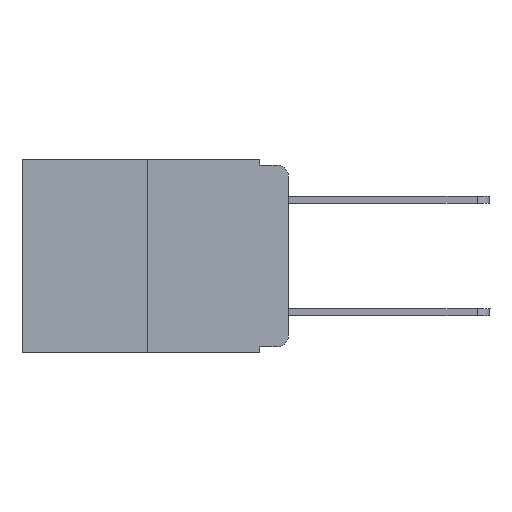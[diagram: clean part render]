
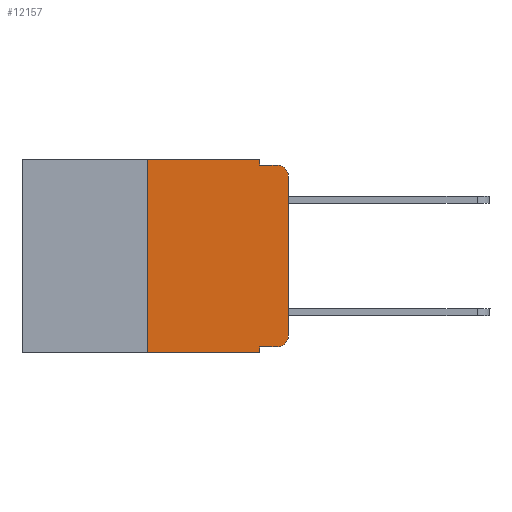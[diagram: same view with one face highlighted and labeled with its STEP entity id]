
A CAD part, left-side view. The second image highlights one B-rep face of the part: STEP entity #12157.
In plain terms, the highlighted planar face has unit normal (-1, 0, 0).
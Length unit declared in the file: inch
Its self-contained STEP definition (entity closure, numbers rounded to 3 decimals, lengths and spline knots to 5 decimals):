
#166 = LINE ( 'NONE', #14627, #7248 ) ;
#282 = EDGE_CURVE ( 'NONE', #3871, #5701, #5324, .T. ) ;
#373 = CARTESIAN_POINT ( 'NONE',  ( 0., 0.02, -0.313 ) ) ;
#478 = ORIENTED_EDGE ( 'NONE', *, *, #15215, .T. ) ;
#643 = VECTOR ( 'NONE', #9150, 39.37008 ) ;
#799 = DIRECTION ( 'NONE',  ( 0., 0., -1. ) ) ;
#820 = VERTEX_POINT ( 'NONE', #844 ) ;
#844 = CARTESIAN_POINT ( 'NONE',  ( 0., 0.02, -0.333 ) ) ;
#1194 = EDGE_CURVE ( 'NONE', #10381, #2462, #6404, .T. ) ;
#1381 = VERTEX_POINT ( 'NONE', #11010 ) ;
#1392 = ORIENTED_EDGE ( 'NONE', *, *, #11559, .T. ) ;
#1695 = DIRECTION ( 'NONE',  ( 0., 0., -1. ) ) ;
#1762 = VECTOR ( 'NONE', #799, 39.37008 ) ;
#2462 = VERTEX_POINT ( 'NONE', #12397 ) ;
#2502 = DIRECTION ( 'NONE',  ( 1., 0., 0. ) ) ;
#2758 = VERTEX_POINT ( 'NONE', #7510 ) ;
#2884 = CARTESIAN_POINT ( 'NONE',  ( 0., 0.051, 0. ) ) ;
#3028 = CARTESIAN_POINT ( 'NONE',  ( 0., 0.25, 0. ) ) ;
#3035 = CARTESIAN_POINT ( 'NONE',  ( 0., 0.02, -0.01 ) ) ;
#3100 = ORIENTED_EDGE ( 'NONE', *, *, #6658, .T. ) ;
#3135 = LINE ( 'NONE', #6988, #15276 ) ;
#3288 = ORIENTED_EDGE ( 'NONE', *, *, #10688, .F. ) ;
#3562 = VECTOR ( 'NONE', #14910, 39.37008 ) ;
#3756 = ORIENTED_EDGE ( 'NONE', *, *, #14790, .F. ) ;
#3871 = VERTEX_POINT ( 'NONE', #12331 ) ;
#4253 = AXIS2_PLACEMENT_3D ( 'NONE', #14451, #2502, #7300 ) ;
#4347 = LINE ( 'NONE', #11509, #643 ) ;
#5076 = DIRECTION ( 'NONE',  ( 0., 0., 1. ) ) ;
#5151 = CARTESIAN_POINT ( 'NONE',  ( 0., 0.051, -0.333 ) ) ;
#5265 = ORIENTED_EDGE ( 'NONE', *, *, #10844, .F. ) ;
#5324 = LINE ( 'NONE', #10128, #11529 ) ;
#5701 = VERTEX_POINT ( 'NONE', #3035 ) ;
#5727 = EDGE_CURVE ( 'NONE', #8226, #2462, #4347, .T. ) ;
#6082 = EDGE_CURVE ( 'NONE', #2758, #5701, #9935, .T. ) ;
#6310 = DIRECTION ( 'NONE',  ( -1., 0., 0. ) ) ;
#6392 = DIRECTION ( 'NONE',  ( 0., 0., -1. ) ) ;
#6404 = LINE ( 'NONE', #13942, #1762 ) ;
#6646 = EDGE_LOOP ( 'NONE', ( #1392, #10962, #12667, #5265, #3756, #3288, #8775, #9556, #3100, #478 ) ) ;
#6658 = EDGE_CURVE ( 'NONE', #10381, #820, #3135, .T. ) ;
#6817 = DIRECTION ( 'NONE',  ( 0., -1., 0. ) ) ;
#6988 = CARTESIAN_POINT ( 'NONE',  ( 0., 0.051, -0.333 ) ) ;
#7248 = VECTOR ( 'NONE', #5076, 39.37008 ) ;
#7300 = DIRECTION ( 'NONE',  ( 0., 0., -1. ) ) ;
#7455 = CARTESIAN_POINT ( 'NONE',  ( 0., 0.25, 0. ) ) ;
#7510 = CARTESIAN_POINT ( 'NONE',  ( 0., 0., -0.03 ) ) ;
#8106 = AXIS2_PLACEMENT_3D ( 'NONE', #373, #9941, #1695 ) ;
#8226 = VERTEX_POINT ( 'NONE', #14887 ) ;
#8463 = LINE ( 'NONE', #7455, #14332 ) ;
#8548 = VERTEX_POINT ( 'NONE', #11387 ) ;
#8775 = ORIENTED_EDGE ( 'NONE', *, *, #5727, .T. ) ;
#8951 = CARTESIAN_POINT ( 'NONE',  ( 0., 0.473, 0. ) ) ;
#9150 = DIRECTION ( 'NONE',  ( 0., -1., 0. ) ) ;
#9556 = ORIENTED_EDGE ( 'NONE', *, *, #1194, .F. ) ;
#9631 = PLANE ( 'NONE',  #4253 ) ;
#9705 = AXIS2_PLACEMENT_3D ( 'NONE', #12301, #6310, #6392 ) ;
#9935 = CIRCLE ( 'NONE', #9705, 0.02 ) ;
#9941 = DIRECTION ( 'NONE',  ( -1., 0., 0. ) ) ;
#10128 = CARTESIAN_POINT ( 'NONE',  ( 0., 0.051, -0.01 ) ) ;
#10381 = VERTEX_POINT ( 'NONE', #5151 ) ;
#10688 = EDGE_CURVE ( 'NONE', #8226, #12285, #8463, .T. ) ;
#10844 = EDGE_CURVE ( 'NONE', #8548, #3871, #14760, .T. ) ;
#10962 = ORIENTED_EDGE ( 'NONE', *, *, #6082, .T. ) ;
#11010 = CARTESIAN_POINT ( 'NONE',  ( 0., 0., -0.313 ) ) ;
#11314 = DIRECTION ( 'NONE',  ( 0., -1., 0. ) ) ;
#11387 = CARTESIAN_POINT ( 'NONE',  ( 0., 0.051, 0. ) ) ;
#11509 = CARTESIAN_POINT ( 'NONE',  ( 0., 0.473, -0.343 ) ) ;
#11529 = VECTOR ( 'NONE', #11314, 39.37008 ) ;
#11559 = EDGE_CURVE ( 'NONE', #1381, #2758, #166, .T. ) ;
#12157 = ADVANCED_FACE ( 'NONE', ( #12161 ), #9631, .F. ) ;
#12161 = FACE_OUTER_BOUND ( 'NONE', #6646, .T. ) ;
#12236 = DIRECTION ( 'NONE',  ( 0., 0., 1. ) ) ;
#12285 = VERTEX_POINT ( 'NONE', #3028 ) ;
#12301 = CARTESIAN_POINT ( 'NONE',  ( 0., 0.02, -0.03 ) ) ;
#12331 = CARTESIAN_POINT ( 'NONE',  ( 0., 0.051, -0.01 ) ) ;
#12397 = CARTESIAN_POINT ( 'NONE',  ( 0., 0.051, -0.343 ) ) ;
#12418 = DIRECTION ( 'NONE',  ( 0., -1., 0. ) ) ;
#12653 = VECTOR ( 'NONE', #12418, 39.37008 ) ;
#12667 = ORIENTED_EDGE ( 'NONE', *, *, #282, .F. ) ;
#12921 = CIRCLE ( 'NONE', #8106, 0.02 ) ;
#13595 = LINE ( 'NONE', #8951, #12653 ) ;
#13942 = CARTESIAN_POINT ( 'NONE',  ( 0., 0.051, 0. ) ) ;
#14332 = VECTOR ( 'NONE', #12236, 39.37008 ) ;
#14451 = CARTESIAN_POINT ( 'NONE',  ( 0., 0.473, 0. ) ) ;
#14627 = CARTESIAN_POINT ( 'NONE',  ( 0., 0., 0. ) ) ;
#14760 = LINE ( 'NONE', #2884, #3562 ) ;
#14790 = EDGE_CURVE ( 'NONE', #12285, #8548, #13595, .T. ) ;
#14887 = CARTESIAN_POINT ( 'NONE',  ( 0., 0.25, -0.343 ) ) ;
#14910 = DIRECTION ( 'NONE',  ( 0., 0., -1. ) ) ;
#15215 = EDGE_CURVE ( 'NONE', #820, #1381, #12921, .T. ) ;
#15276 = VECTOR ( 'NONE', #6817, 39.37008 ) ;
